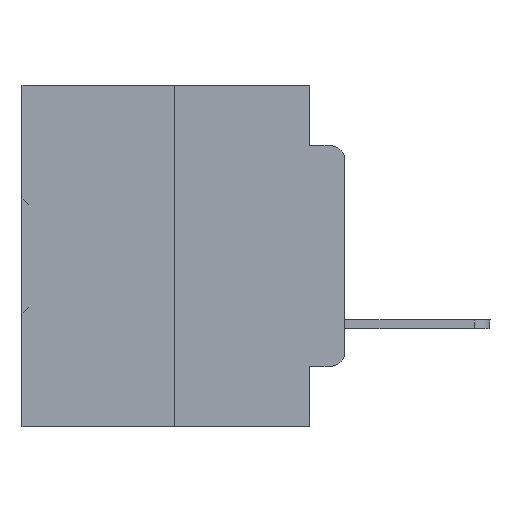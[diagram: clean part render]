
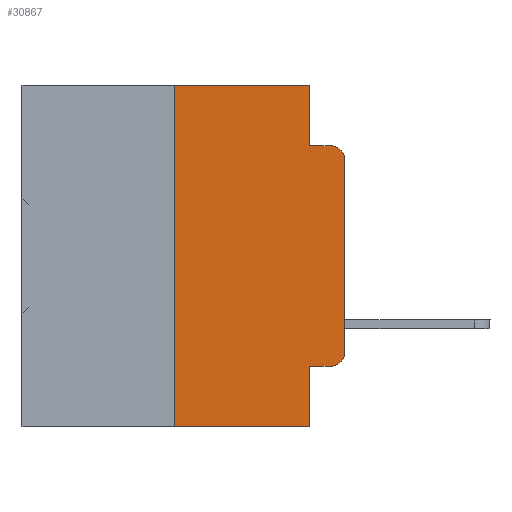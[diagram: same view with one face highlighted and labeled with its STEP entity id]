
A CAD part, left-side view. The second image highlights one B-rep face of the part: STEP entity #30867.
In plain terms, the highlighted planar face has unit normal (-1, 0, 0).
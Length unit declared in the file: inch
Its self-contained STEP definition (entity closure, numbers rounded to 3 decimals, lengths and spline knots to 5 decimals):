
#53 = CARTESIAN_POINT ( 'NONE',  ( 0., 0.051, -0.0885 ) ) ;
#858 = ORIENTED_EDGE ( 'NONE', *, *, #31568, .F. ) ;
#1004 = VECTOR ( 'NONE', #9053, 39.37008 ) ;
#1435 = CARTESIAN_POINT ( 'NONE',  ( 0., 0., -0.1085 ) ) ;
#1652 = AXIS2_PLACEMENT_3D ( 'NONE', #34703, #26414, #29429 ) ;
#1777 = CARTESIAN_POINT ( 'NONE',  ( 0., 0.051, 0. ) ) ;
#2141 = CARTESIAN_POINT ( 'NONE',  ( 0., 0.473, -0.5 ) ) ;
#2608 = VECTOR ( 'NONE', #8791, 39.37008 ) ;
#2797 = LINE ( 'NONE', #5061, #21918 ) ;
#2936 = LINE ( 'NONE', #17221, #2608 ) ;
#3535 = VECTOR ( 'NONE', #28349, 39.37008 ) ;
#3673 = ORIENTED_EDGE ( 'NONE', *, *, #12936, .F. ) ;
#4462 = VERTEX_POINT ( 'NONE', #10123 ) ;
#4826 = CARTESIAN_POINT ( 'NONE',  ( 0., 0.051, -0.0885 ) ) ;
#5061 = CARTESIAN_POINT ( 'NONE',  ( 0., 0.051, 0. ) ) ;
#5427 = CARTESIAN_POINT ( 'NONE',  ( 0., 0.051, 0. ) ) ;
#5534 = VERTEX_POINT ( 'NONE', #1435 ) ;
#5571 = CARTESIAN_POINT ( 'NONE',  ( 0., 0.02, -0.1085 ) ) ;
#5696 = VECTOR ( 'NONE', #10836, 39.37008 ) ;
#6317 = DIRECTION ( 'NONE',  ( -1., 0., 0. ) ) ;
#7089 = EDGE_CURVE ( 'NONE', #5534, #13923, #12894, .T. ) ;
#7123 = VECTOR ( 'NONE', #35632, 39.37008 ) ;
#7265 = LINE ( 'NONE', #18339, #7123 ) ;
#7339 = EDGE_CURVE ( 'NONE', #4462, #28136, #16239, .T. ) ;
#7552 = CARTESIAN_POINT ( 'NONE',  ( 0., 0., -0.3915 ) ) ;
#8397 = CIRCLE ( 'NONE', #10207, 0.02 ) ;
#8791 = DIRECTION ( 'NONE',  ( 0., -1., 0. ) ) ;
#9053 = DIRECTION ( 'NONE',  ( 0., -1., 0. ) ) ;
#9507 = ORIENTED_EDGE ( 'NONE', *, *, #27338, .F. ) ;
#10123 = CARTESIAN_POINT ( 'NONE',  ( 0., 0.25, -0.5 ) ) ;
#10207 = AXIS2_PLACEMENT_3D ( 'NONE', #21755, #13305, #36415 ) ;
#10836 = DIRECTION ( 'NONE',  ( 0., -1., 0. ) ) ;
#10933 = DIRECTION ( 'NONE',  ( 0., 0., -1. ) ) ;
#11688 = LINE ( 'NONE', #28768, #1004 ) ;
#12330 = VERTEX_POINT ( 'NONE', #33323 ) ;
#12894 = CIRCLE ( 'NONE', #35696, 0.02 ) ;
#12936 = EDGE_CURVE ( 'NONE', #12330, #27824, #2936, .T. ) ;
#13305 = DIRECTION ( 'NONE',  ( -1., 0., 0. ) ) ;
#13877 = LINE ( 'NONE', #4826, #32150 ) ;
#13923 = VERTEX_POINT ( 'NONE', #29712 ) ;
#14234 = EDGE_CURVE ( 'NONE', #27824, #32626, #2797, .T. ) ;
#16239 = LINE ( 'NONE', #2141, #5696 ) ;
#17062 = CARTESIAN_POINT ( 'NONE',  ( 0., 0.02, -0.4115 ) ) ;
#17221 = CARTESIAN_POINT ( 'NONE',  ( 0., 0.473, 0. ) ) ;
#18126 = FACE_OUTER_BOUND ( 'NONE', #31900, .T. ) ;
#18194 = VERTEX_POINT ( 'NONE', #7552 ) ;
#18339 = CARTESIAN_POINT ( 'NONE',  ( 0., 0., 0. ) ) ;
#19616 = VECTOR ( 'NONE', #28012, 39.37008 ) ;
#19788 = ORIENTED_EDGE ( 'NONE', *, *, #7339, .T. ) ;
#20825 = EDGE_CURVE ( 'NONE', #18194, #5534, #7265, .T. ) ;
#21755 = CARTESIAN_POINT ( 'NONE',  ( 0., 0.02, -0.3915 ) ) ;
#21918 = VECTOR ( 'NONE', #10933, 39.37008 ) ;
#23782 = ORIENTED_EDGE ( 'NONE', *, *, #29903, .T. ) ;
#23954 = PLANE ( 'NONE',  #1652 ) ;
#24294 = ORIENTED_EDGE ( 'NONE', *, *, #20825, .T. ) ;
#24476 = ORIENTED_EDGE ( 'NONE', *, *, #31907, .T. ) ;
#24637 = LINE ( 'NONE', #28204, #19616 ) ;
#25667 = DIRECTION ( 'NONE',  ( 0., 0., -1. ) ) ;
#26414 = DIRECTION ( 'NONE',  ( 1., 0., 0. ) ) ;
#26562 = CARTESIAN_POINT ( 'NONE',  ( 0., 0.051, -0.5 ) ) ;
#27338 = EDGE_CURVE ( 'NONE', #32626, #13923, #13877, .T. ) ;
#27824 = VERTEX_POINT ( 'NONE', #1777 ) ;
#28012 = DIRECTION ( 'NONE',  ( 0., 0., 1. ) ) ;
#28136 = VERTEX_POINT ( 'NONE', #26562 ) ;
#28204 = CARTESIAN_POINT ( 'NONE',  ( 0., 0.25, 0. ) ) ;
#28349 = DIRECTION ( 'NONE',  ( 0., 0., -1. ) ) ;
#28768 = CARTESIAN_POINT ( 'NONE',  ( 0., 0.051, -0.4115 ) ) ;
#29429 = DIRECTION ( 'NONE',  ( 0., 0., -1. ) ) ;
#29712 = CARTESIAN_POINT ( 'NONE',  ( 0., 0.02, -0.0885 ) ) ;
#29800 = EDGE_CURVE ( 'NONE', #4462, #12330, #24637, .T. ) ;
#29903 = EDGE_CURVE ( 'NONE', #36476, #31610, #11688, .T. ) ;
#30084 = ORIENTED_EDGE ( 'NONE', *, *, #29800, .F. ) ;
#30826 = ORIENTED_EDGE ( 'NONE', *, *, #14234, .F. ) ;
#30867 = ADVANCED_FACE ( 'NONE', ( #18126 ), #23954, .F. ) ;
#31568 = EDGE_CURVE ( 'NONE', #36476, #28136, #36830, .T. ) ;
#31610 = VERTEX_POINT ( 'NONE', #17062 ) ;
#31900 = EDGE_LOOP ( 'NONE', ( #24294, #34355, #9507, #30826, #3673, #30084, #19788, #858, #23782, #24476 ) ) ;
#31907 = EDGE_CURVE ( 'NONE', #31610, #18194, #8397, .T. ) ;
#32150 = VECTOR ( 'NONE', #36236, 39.37008 ) ;
#32626 = VERTEX_POINT ( 'NONE', #53 ) ;
#33323 = CARTESIAN_POINT ( 'NONE',  ( 0., 0.25, 0. ) ) ;
#33564 = CARTESIAN_POINT ( 'NONE',  ( 0., 0.051, -0.4115 ) ) ;
#34355 = ORIENTED_EDGE ( 'NONE', *, *, #7089, .T. ) ;
#34703 = CARTESIAN_POINT ( 'NONE',  ( 0., 0.473, 0. ) ) ;
#35632 = DIRECTION ( 'NONE',  ( 0., 0., 1. ) ) ;
#35696 = AXIS2_PLACEMENT_3D ( 'NONE', #5571, #6317, #25667 ) ;
#36236 = DIRECTION ( 'NONE',  ( 0., -1., 0. ) ) ;
#36415 = DIRECTION ( 'NONE',  ( 0., 0., -1. ) ) ;
#36476 = VERTEX_POINT ( 'NONE', #33564 ) ;
#36830 = LINE ( 'NONE', #5427, #3535 ) ;
